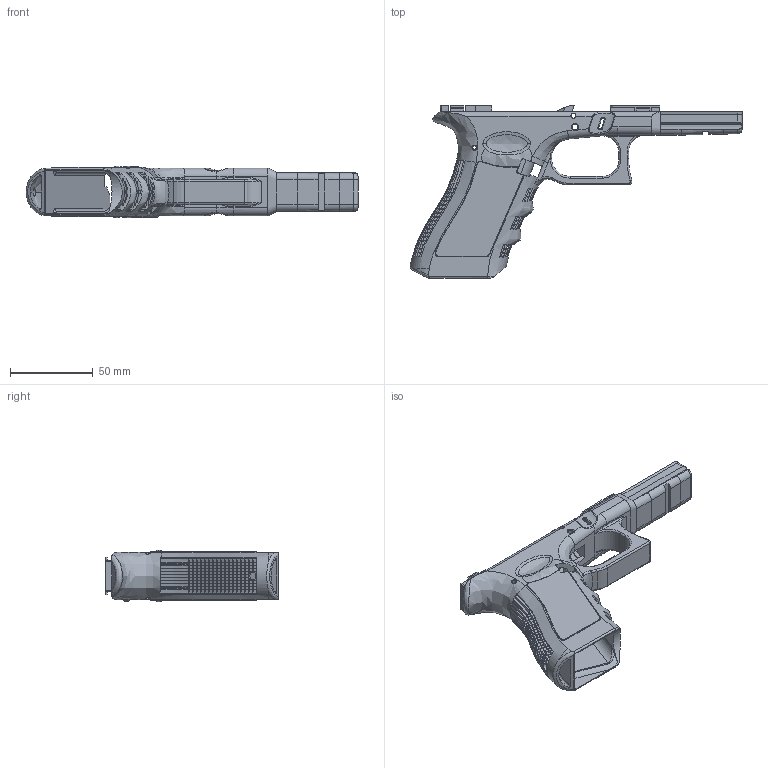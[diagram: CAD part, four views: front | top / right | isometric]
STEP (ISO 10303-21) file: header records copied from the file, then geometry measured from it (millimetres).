
FILE_DESCRIPTION(/* description */ (''),/* implementation_level */ '2;1');
FILE_NAME(/* name */ 'Glock_frame.step',/* time_stamp */ '2020-09-03T15:08:54-04:00',/* author */ (''),/* organization */ (''),/* preprocessor_version */ 'ST-DEVELOPER v18.1',/* originating_system */ 'Autodesk Translation Framework v9.3.0.1241',/* authorisation */ '');
FILE_SCHEMA (('AUTOMOTIVE_DESIGN { 1 0 10303 214 3 1 1 }'));
Products named in the file (1): Glock_frame
Bounding box: 201.04 x 104.61 x 31.35 mm (x, y, z)
Volume: 81091.9 mm3; surface area: 51180 mm2
Topology: 1 solids, 1 shells, 1841 faces, 4430 edges, 2577 vertices
Faces by surface type: plane 1085, bspline 553, cylinder 154, torus 39, sphere 8, cone 2
Full cylindrical faces by diameter (mm): 2.286 x2, 3 x2, 3.5 x2, 4.978 x1
Entity records: 110749 total; most frequent: CARTESIAN_POINT 73539, ORIENTED_EDGE 8842, DIRECTION 5709, EDGE_CURVE 4421, VERTEX_POINT 2577, LINE 2067, VECTOR 2067, EDGE_LOOP 1866
